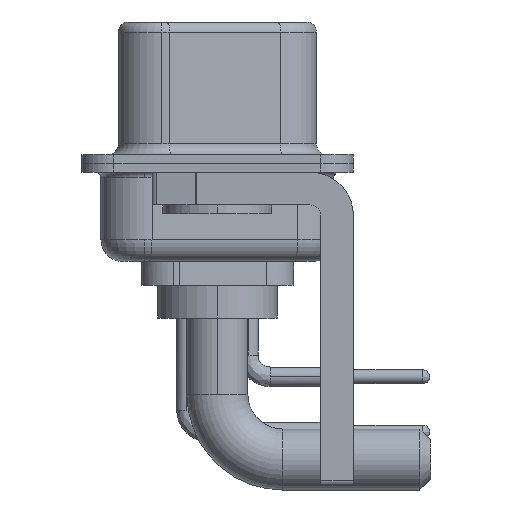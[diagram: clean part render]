
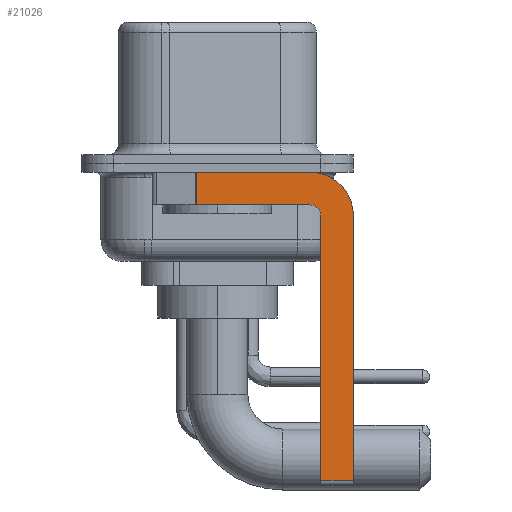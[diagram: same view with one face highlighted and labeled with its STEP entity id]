
A CAD part, left-side view. The second image highlights one B-rep face of the part: STEP entity #21026.
In plain terms, the highlighted planar face has unit normal (-1, 0, 0).
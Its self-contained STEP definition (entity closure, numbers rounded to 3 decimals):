
#117 = CARTESIAN_POINT ( 'NONE',  ( -2.9, -6.25, -2.4 ) ) ;
#181 = ORIENTED_EDGE ( 'NONE', *, *, #10487, .F. ) ;
#210 = DIRECTION ( 'NONE',  ( 0., 1., 0. ) ) ;
#343 = VECTOR ( 'NONE', #16428, 1000. ) ;
#423 = CARTESIAN_POINT ( 'NONE',  ( -2.9, -6.25, -14.55 ) ) ;
#842 = CARTESIAN_POINT ( 'NONE',  ( -2.9, -4.25, -1.9 ) ) ;
#1721 = VECTOR ( 'NONE', #14112, 1000. ) ;
#2343 = ORIENTED_EDGE ( 'NONE', *, *, #17177, .F. ) ;
#2562 = ORIENTED_EDGE ( 'NONE', *, *, #14795, .F. ) ;
#2643 = CARTESIAN_POINT ( 'NONE',  ( -2.9, 3., -0.4 ) ) ;
#2725 = VECTOR ( 'NONE', #7860, 1000. ) ;
#2993 = CARTESIAN_POINT ( 'NONE',  ( -2.9, -4.25, -0.4 ) ) ;
#3148 = CARTESIAN_POINT ( 'NONE',  ( -2.9, 0.978, -1.9 ) ) ;
#3368 = CIRCLE ( 'NONE', #24224, 2. ) ;
#3457 = VERTEX_POINT ( 'NONE', #842 ) ;
#3929 = FACE_OUTER_BOUND ( 'NONE', #18936, .T. ) ;
#3994 = CARTESIAN_POINT ( 'NONE',  ( -2.9, -4.25, -2.4 ) ) ;
#5121 = DIRECTION ( 'NONE',  ( 0., 0., 1. ) ) ;
#5418 = CARTESIAN_POINT ( 'NONE',  ( -2.9, -4.75, -2.4 ) ) ;
#5451 = LINE ( 'NONE', #12482, #22461 ) ;
#5883 = CARTESIAN_POINT ( 'NONE',  ( -2.9, -4.25, -14.55 ) ) ;
#6389 = EDGE_CURVE ( 'NONE', #19346, #20806, #20556, .T. ) ;
#7620 = DIRECTION ( 'NONE',  ( 1., 0., 0. ) ) ;
#7674 = DIRECTION ( 'NONE',  ( 0., 0., -1. ) ) ;
#7860 = DIRECTION ( 'NONE',  ( 0., -1., 0. ) ) ;
#8183 = LINE ( 'NONE', #2643, #1721 ) ;
#8942 = ORIENTED_EDGE ( 'NONE', *, *, #6389, .T. ) ;
#9492 = CARTESIAN_POINT ( 'NONE',  ( -2.9, -4.75, -14.8 ) ) ;
#9529 = CIRCLE ( 'NONE', #10698, 0.5 ) ;
#10302 = ORIENTED_EDGE ( 'NONE', *, *, #16028, .F. ) ;
#10487 = EDGE_CURVE ( 'NONE', #12497, #20806, #20349, .T. ) ;
#10698 = AXIS2_PLACEMENT_3D ( 'NONE', #14634, #16342, #5121 ) ;
#12482 = CARTESIAN_POINT ( 'NONE',  ( -2.9, 0.978, -1.9 ) ) ;
#12497 = VERTEX_POINT ( 'NONE', #117 ) ;
#12616 = DIRECTION ( 'NONE',  ( 0., 0., -1. ) ) ;
#13302 = VECTOR ( 'NONE', #17006, 1000. ) ;
#13843 = VERTEX_POINT ( 'NONE', #2993 ) ;
#13929 = EDGE_CURVE ( 'NONE', #22057, #23081, #5451, .T. ) ;
#14066 = CARTESIAN_POINT ( 'NONE',  ( -2.9, -4.75, -14.55 ) ) ;
#14112 = DIRECTION ( 'NONE',  ( 0., -1., 0. ) ) ;
#14407 = VERTEX_POINT ( 'NONE', #5418 ) ;
#14462 = DIRECTION ( 'NONE',  ( 0., 0., -1. ) ) ;
#14634 = CARTESIAN_POINT ( 'NONE',  ( -2.9, -4.25, -2.4 ) ) ;
#14715 = CARTESIAN_POINT ( 'NONE',  ( -2.9, -6.25, -2.4 ) ) ;
#14795 = EDGE_CURVE ( 'NONE', #14407, #3457, #9529, .T. ) ;
#15349 = DIRECTION ( 'NONE',  ( 1., 0., 0. ) ) ;
#16028 = EDGE_CURVE ( 'NONE', #22057, #13843, #8183, .T. ) ;
#16342 = DIRECTION ( 'NONE',  ( -1., 0., 0. ) ) ;
#16428 = DIRECTION ( 'NONE',  ( 0., 0., -1. ) ) ;
#16546 = CARTESIAN_POINT ( 'NONE',  ( -2.9, -4.25, -2.4 ) ) ;
#16595 = ORIENTED_EDGE ( 'NONE', *, *, #20813, .F. ) ;
#17006 = DIRECTION ( 'NONE',  ( 0., 0., 1. ) ) ;
#17177 = EDGE_CURVE ( 'NONE', #3457, #23081, #22269, .T. ) ;
#17423 = CARTESIAN_POINT ( 'NONE',  ( -2.9, 0.978, -0.4 ) ) ;
#17930 = AXIS2_PLACEMENT_3D ( 'NONE', #16546, #7620, #14462 ) ;
#18936 = EDGE_LOOP ( 'NONE', ( #10302, #24035, #2343, #2562, #23704, #8942, #181, #16595 ) ) ;
#18956 = PLANE ( 'NONE',  #17930 ) ;
#19346 = VERTEX_POINT ( 'NONE', #14066 ) ;
#20349 = LINE ( 'NONE', #14715, #343 ) ;
#20556 = LINE ( 'NONE', #5883, #2725 ) ;
#20806 = VERTEX_POINT ( 'NONE', #423 ) ;
#20813 = EDGE_CURVE ( 'NONE', #13843, #12497, #3368, .T. ) ;
#21026 = ADVANCED_FACE ( 'NONE', ( #3929 ), #18956, .F. ) ;
#22057 = VERTEX_POINT ( 'NONE', #17423 ) ;
#22269 = LINE ( 'NONE', #24245, #22574 ) ;
#22461 = VECTOR ( 'NONE', #12616, 1000. ) ;
#22574 = VECTOR ( 'NONE', #210, 1000. ) ;
#22777 = LINE ( 'NONE', #9492, #13302 ) ;
#23005 = EDGE_CURVE ( 'NONE', #19346, #14407, #22777, .T. ) ;
#23081 = VERTEX_POINT ( 'NONE', #3148 ) ;
#23704 = ORIENTED_EDGE ( 'NONE', *, *, #23005, .F. ) ;
#24035 = ORIENTED_EDGE ( 'NONE', *, *, #13929, .T. ) ;
#24224 = AXIS2_PLACEMENT_3D ( 'NONE', #3994, #15349, #7674 ) ;
#24245 = CARTESIAN_POINT ( 'NONE',  ( -2.9, -4.25, -1.9 ) ) ;
